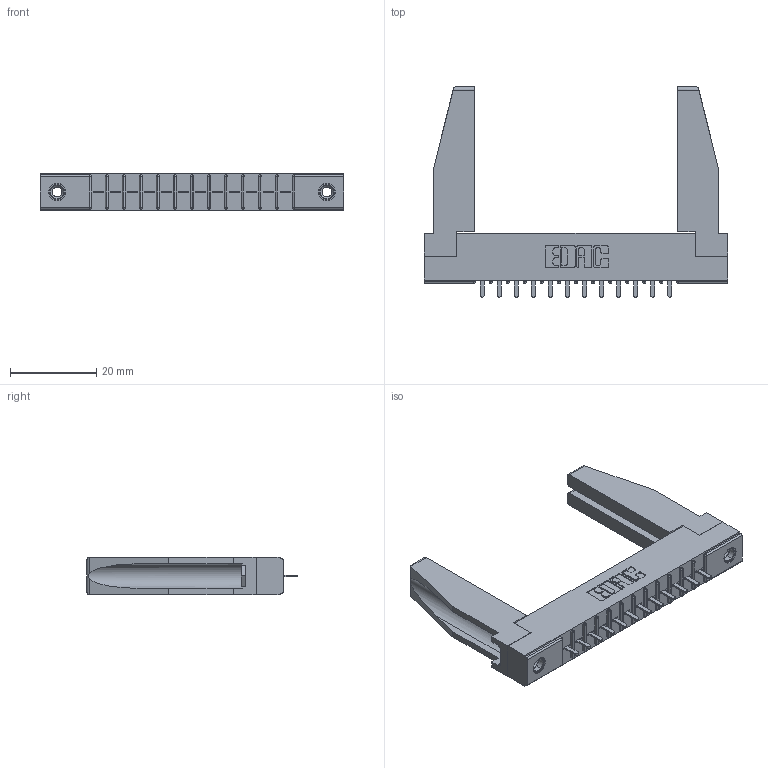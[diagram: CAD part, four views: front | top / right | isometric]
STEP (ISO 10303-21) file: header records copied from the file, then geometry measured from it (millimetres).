
FILE_DESCRIPTION (( 'STEP AP203' ), '1' );
FILE_NAME ('316-012-521-178.STEP', '2018-07-31T00:29:10', ( '' ), ( '' ), 'SwSTEP 2.0', 'SolidWorks 2016', '' );
FILE_SCHEMA (( 'CONFIG_CONTROL_DESIGN' ));
Length unit declared in the file: inch
Products named in the file (5): 316-012-521-178; 306 Part_.156 Dia; 306-290-001_121; 345-250-001_345-250-001-102; 307-220-078
Assembly tree (17 placements, depth 2):
  316-012-521-178
    306 Part_.156 Dia
    306-290-001_121  x12
    345-250-001_345-250-001-102  x2
    307-220-078  x2
Bounding box: 70.56 x 48.92 x 8.71 mm (x, y, z)
Volume: 8763.6 mm3; surface area: 10474.1 mm2
Topology: 17 solids, 17 shells, 1086 faces, 3010 edges, 1932 vertices
Faces by surface type: plane 716, cylinder 306, sphere 48, cone 12, torus 4
Entity records: 17472 total; most frequent: CARTESIAN_POINT 2929, ORIENTED_EDGE 2858, DIRECTION 2843, EDGE_CURVE 1429, VECTOR 1103, LINE 1103, VERTEX_POINT 914, AXIS2_PLACEMENT_3D 870
